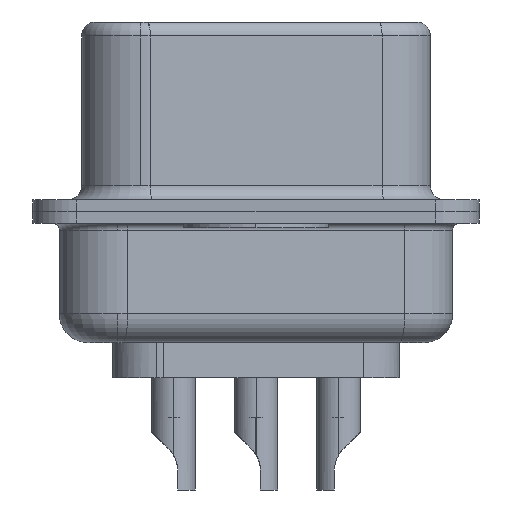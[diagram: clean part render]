
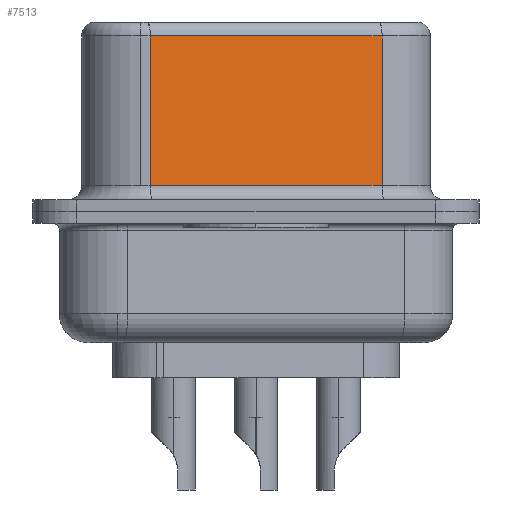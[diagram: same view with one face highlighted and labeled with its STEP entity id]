
A CAD part, left-side view. The second image highlights one B-rep face of the part: STEP entity #7513.
In plain terms, the highlighted planar face has unit normal (-0.985, -0.174, 0).
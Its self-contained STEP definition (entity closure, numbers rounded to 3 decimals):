
#523 = EDGE_CURVE ( 'NONE', #5308, #5395, #18974, .T. ) ;
#1493 = LINE ( 'NONE', #11867, #20447 ) ;
#1732 = DIRECTION ( 'NONE',  ( 0.985, 0.174, 0. ) ) ;
#2599 = ORIENTED_EDGE ( 'NONE', *, *, #11452, .T. ) ;
#3751 = DIRECTION ( 'NONE',  ( 0.174, -0.985, 0. ) ) ;
#4397 = CARTESIAN_POINT ( 'NONE',  ( 3.73, 3.628, 6.52 ) ) ;
#5056 = ORIENTED_EDGE ( 'NONE', *, *, #523, .F. ) ;
#5308 = VERTEX_POINT ( 'NONE', #27124 ) ;
#5395 = VERTEX_POINT ( 'NONE', #27397 ) ;
#6757 = ORIENTED_EDGE ( 'NONE', *, *, #20122, .T. ) ;
#7513 = ADVANCED_FACE ( 'NONE', ( #14782 ), #25160, .F. ) ;
#8592 = DIRECTION ( 'NONE',  ( 0., 0., -1. ) ) ;
#8652 = LINE ( 'NONE', #16947, #17077 ) ;
#9826 = VERTEX_POINT ( 'NONE', #13862 ) ;
#10559 = CARTESIAN_POINT ( 'NONE',  ( 5.132, -4.322, 6.52 ) ) ;
#11452 = EDGE_CURVE ( 'NONE', #9826, #5395, #1493, .T. ) ;
#11867 = CARTESIAN_POINT ( 'NONE',  ( 5.132, -4.322, 0.9 ) ) ;
#13666 = ORIENTED_EDGE ( 'NONE', *, *, #22282, .T. ) ;
#13862 = CARTESIAN_POINT ( 'NONE',  ( 3.73, 3.628, 0.9 ) ) ;
#14782 = FACE_OUTER_BOUND ( 'NONE', #19988, .T. ) ;
#16003 = VERTEX_POINT ( 'NONE', #18538 ) ;
#16737 = AXIS2_PLACEMENT_3D ( 'NONE', #10559, #1732, #25438 ) ;
#16947 = CARTESIAN_POINT ( 'NONE',  ( 5.132, -4.322, 6.02 ) ) ;
#17077 = VECTOR ( 'NONE', #25499, 1000. ) ;
#17786 = VECTOR ( 'NONE', #23607, 1000. ) ;
#18538 = CARTESIAN_POINT ( 'NONE',  ( 3.73, 3.628, 6.02 ) ) ;
#18974 = LINE ( 'NONE', #27535, #17786 ) ;
#19988 = EDGE_LOOP ( 'NONE', ( #5056, #6757, #13666, #2599 ) ) ;
#20122 = EDGE_CURVE ( 'NONE', #5308, #16003, #8652, .T. ) ;
#20447 = VECTOR ( 'NONE', #3751, 1000. ) ;
#22282 = EDGE_CURVE ( 'NONE', #16003, #9826, #27259, .T. ) ;
#23607 = DIRECTION ( 'NONE',  ( 0., 0., -1. ) ) ;
#25160 = PLANE ( 'NONE',  #16737 ) ;
#25438 = DIRECTION ( 'NONE',  ( -0.174, 0.985, 0. ) ) ;
#25499 = DIRECTION ( 'NONE',  ( -0.174, 0.985, 0. ) ) ;
#25684 = VECTOR ( 'NONE', #8592, 1000. ) ;
#27124 = CARTESIAN_POINT ( 'NONE',  ( 5.132, -4.322, 6.02 ) ) ;
#27259 = LINE ( 'NONE', #4397, #25684 ) ;
#27397 = CARTESIAN_POINT ( 'NONE',  ( 5.132, -4.322, 0.9 ) ) ;
#27535 = CARTESIAN_POINT ( 'NONE',  ( 5.132, -4.322, 6.52 ) ) ;
